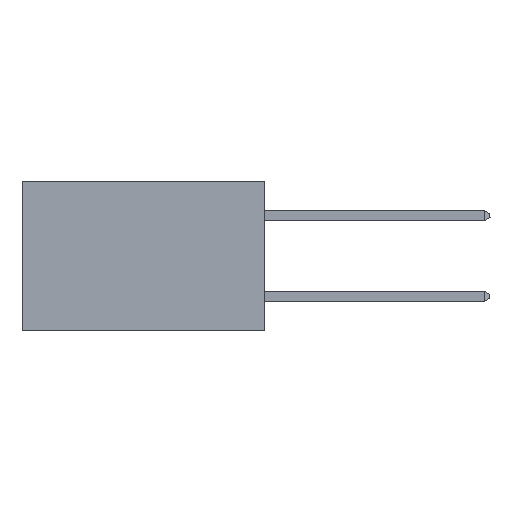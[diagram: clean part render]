
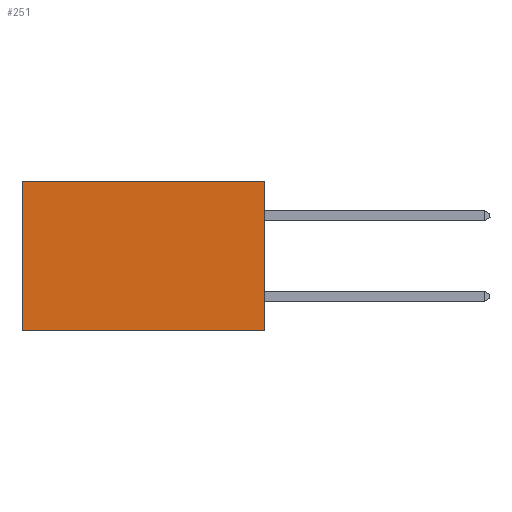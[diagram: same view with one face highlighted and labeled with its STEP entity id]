
A CAD part, left-side view. The second image highlights one B-rep face of the part: STEP entity #251.
In plain terms, the highlighted planar face has unit normal (-1, 0, 0).
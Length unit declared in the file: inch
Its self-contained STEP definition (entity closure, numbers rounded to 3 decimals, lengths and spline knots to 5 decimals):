
#70 = VERTEX_POINT ( 'NONE', #8944 ) ;
#127 = PLANE ( 'NONE',  #5546 ) ;
#251 = ADVANCED_FACE ( 'NONE', ( #2257 ), #127, .F. ) ;
#582 = VECTOR ( 'NONE', #4346, 39.37008 ) ;
#646 = EDGE_LOOP ( 'NONE', ( #2253, #1563, #1471, #2587 ) ) ;
#668 = LINE ( 'NONE', #5770, #6393 ) ;
#1278 = LINE ( 'NONE', #5846, #582 ) ;
#1298 = DIRECTION ( 'NONE',  ( 0., 0., -1. ) ) ;
#1460 = CARTESIAN_POINT ( 'NONE',  ( 0.298, 0.6, -0.37 ) ) ;
#1471 = ORIENTED_EDGE ( 'NONE', *, *, #4747, .F. ) ;
#1563 = ORIENTED_EDGE ( 'NONE', *, *, #8204, .F. ) ;
#1673 = DIRECTION ( 'NONE',  ( 0., 0., -1. ) ) ;
#1938 = DIRECTION ( 'NONE',  ( 0., 1., 0. ) ) ;
#2253 = ORIENTED_EDGE ( 'NONE', *, *, #9289, .T. ) ;
#2257 = FACE_OUTER_BOUND ( 'NONE', #646, .T. ) ;
#2483 = DIRECTION ( 'NONE',  ( 1., 0., 0. ) ) ;
#2587 = ORIENTED_EDGE ( 'NONE', *, *, #3808, .T. ) ;
#3177 = LINE ( 'NONE', #4492, #7525 ) ;
#3354 = VERTEX_POINT ( 'NONE', #1460 ) ;
#3808 = EDGE_CURVE ( 'NONE', #70, #7355, #4885, .T. ) ;
#4346 = DIRECTION ( 'NONE',  ( 0., 0., -1. ) ) ;
#4492 = CARTESIAN_POINT ( 'NONE',  ( 0.298, 0., -0.37 ) ) ;
#4517 = DIRECTION ( 'NONE',  ( 0., 1., 0. ) ) ;
#4747 = EDGE_CURVE ( 'NONE', #70, #7949, #668, .T. ) ;
#4885 = LINE ( 'NONE', #5035, #8899 ) ;
#5035 = CARTESIAN_POINT ( 'NONE',  ( 0.298, 0., 0. ) ) ;
#5076 = CARTESIAN_POINT ( 'NONE',  ( 0.298, 0.6, 0. ) ) ;
#5379 = CARTESIAN_POINT ( 'NONE',  ( 0.298, 0., 0. ) ) ;
#5546 = AXIS2_PLACEMENT_3D ( 'NONE', #5379, #2483, #1673 ) ;
#5770 = CARTESIAN_POINT ( 'NONE',  ( 0.298, 0., 0. ) ) ;
#5846 = CARTESIAN_POINT ( 'NONE',  ( 0.298, 0.6, 0. ) ) ;
#6393 = VECTOR ( 'NONE', #1298, 39.37008 ) ;
#6507 = CARTESIAN_POINT ( 'NONE',  ( 0.298, 0., -0.37 ) ) ;
#7355 = VERTEX_POINT ( 'NONE', #5076 ) ;
#7525 = VECTOR ( 'NONE', #4517, 39.37008 ) ;
#7949 = VERTEX_POINT ( 'NONE', #6507 ) ;
#8204 = EDGE_CURVE ( 'NONE', #7949, #3354, #3177, .T. ) ;
#8899 = VECTOR ( 'NONE', #1938, 39.37008 ) ;
#8944 = CARTESIAN_POINT ( 'NONE',  ( 0.298, 0., 0. ) ) ;
#9289 = EDGE_CURVE ( 'NONE', #7355, #3354, #1278, .T. ) ;
